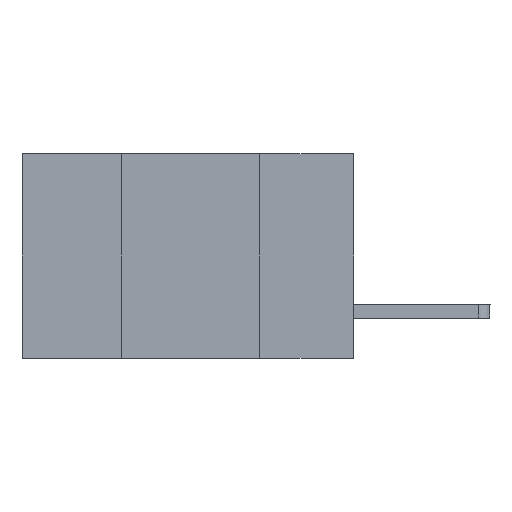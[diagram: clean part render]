
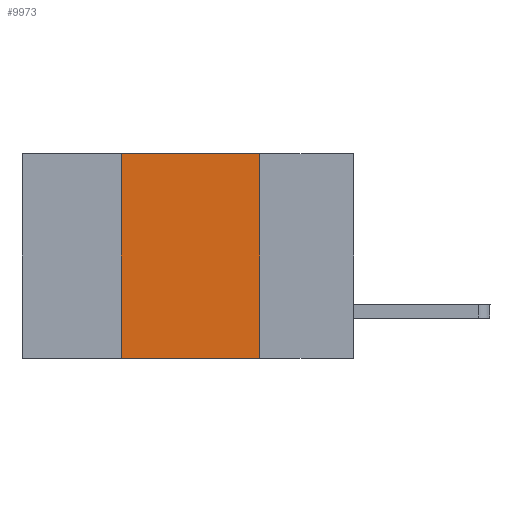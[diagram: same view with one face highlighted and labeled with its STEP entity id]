
A CAD part, left-side view. The second image highlights one B-rep face of the part: STEP entity #9973.
In plain terms, the highlighted planar face has unit normal (-1, 0, 0).
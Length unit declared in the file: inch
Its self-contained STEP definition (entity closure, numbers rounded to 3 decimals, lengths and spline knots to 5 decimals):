
#164 = CARTESIAN_POINT ( 'NONE',  ( 0., 0.42, -0.37 ) ) ;
#179 = VERTEX_POINT ( 'NONE', #2076 ) ;
#285 = LINE ( 'NONE', #1827, #2550 ) ;
#632 = DIRECTION ( 'NONE',  ( 0., 0., 1. ) ) ;
#951 = ORIENTED_EDGE ( 'NONE', *, *, #7132, .T. ) ;
#1827 = CARTESIAN_POINT ( 'NONE',  ( 0., 0.17, 0. ) ) ;
#2066 = VERTEX_POINT ( 'NONE', #164 ) ;
#2076 = CARTESIAN_POINT ( 'NONE',  ( 0., 0.17, -0.37 ) ) ;
#2133 = FACE_OUTER_BOUND ( 'NONE', #6073, .T. ) ;
#2550 = VECTOR ( 'NONE', #5523, 39.37008 ) ;
#2691 = CARTESIAN_POINT ( 'NONE',  ( 0., 0.6, 0. ) ) ;
#2699 = VERTEX_POINT ( 'NONE', #5302 ) ;
#2790 = VERTEX_POINT ( 'NONE', #10982 ) ;
#2843 = EDGE_CURVE ( 'NONE', #2699, #179, #285, .T. ) ;
#3114 = LINE ( 'NONE', #2691, #7411 ) ;
#3404 = DIRECTION ( 'NONE',  ( 0., 0., -1. ) ) ;
#3515 = CARTESIAN_POINT ( 'NONE',  ( 0., 0.42, 0. ) ) ;
#3667 = EDGE_CURVE ( 'NONE', #2790, #2699, #3114, .T. ) ;
#3728 = DIRECTION ( 'NONE',  ( 0., -1., 0. ) ) ;
#3730 = VECTOR ( 'NONE', #3728, 39.37008 ) ;
#4545 = AXIS2_PLACEMENT_3D ( 'NONE', #5169, #8978, #3404 ) ;
#5169 = CARTESIAN_POINT ( 'NONE',  ( 0., 0.6, 0. ) ) ;
#5302 = CARTESIAN_POINT ( 'NONE',  ( 0., 0.17, 0. ) ) ;
#5419 = LINE ( 'NONE', #9243, #3730 ) ;
#5431 = DIRECTION ( 'NONE',  ( 0., -1., 0. ) ) ;
#5523 = DIRECTION ( 'NONE',  ( 0., 0., -1. ) ) ;
#6073 = EDGE_LOOP ( 'NONE', ( #9910, #6077, #10133, #951 ) ) ;
#6077 = ORIENTED_EDGE ( 'NONE', *, *, #3667, .F. ) ;
#7132 = EDGE_CURVE ( 'NONE', #2066, #179, #5419, .T. ) ;
#7411 = VECTOR ( 'NONE', #5431, 39.37008 ) ;
#8403 = EDGE_CURVE ( 'NONE', #2066, #2790, #10795, .T. ) ;
#8797 = VECTOR ( 'NONE', #632, 39.37008 ) ;
#8978 = DIRECTION ( 'NONE',  ( 1., 0., 0. ) ) ;
#9243 = CARTESIAN_POINT ( 'NONE',  ( 0., 0.6, -0.37 ) ) ;
#9910 = ORIENTED_EDGE ( 'NONE', *, *, #2843, .F. ) ;
#9973 = ADVANCED_FACE ( 'NONE', ( #2133 ), #11620, .F. ) ;
#10133 = ORIENTED_EDGE ( 'NONE', *, *, #8403, .F. ) ;
#10795 = LINE ( 'NONE', #3515, #8797 ) ;
#10982 = CARTESIAN_POINT ( 'NONE',  ( 0., 0.42, 0. ) ) ;
#11620 = PLANE ( 'NONE',  #4545 ) ;
